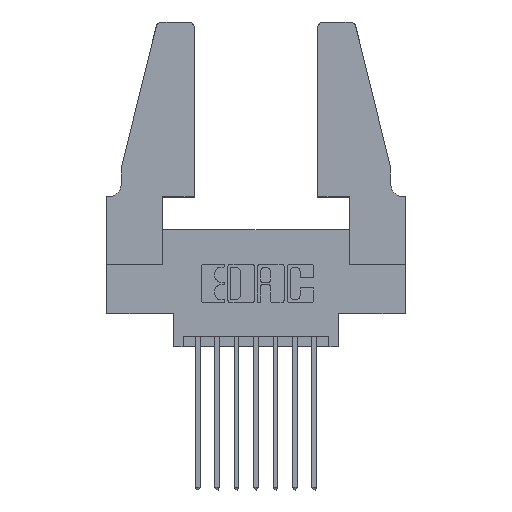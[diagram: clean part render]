
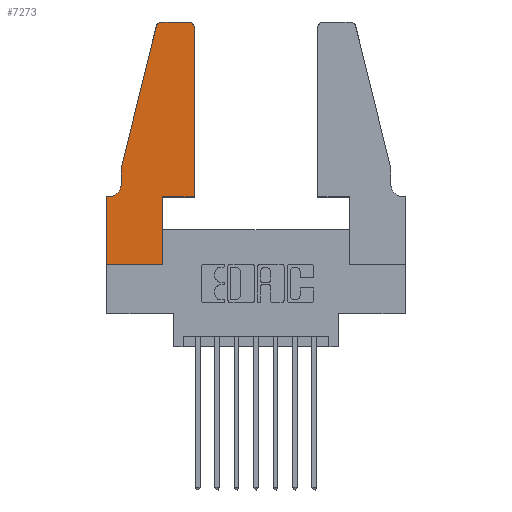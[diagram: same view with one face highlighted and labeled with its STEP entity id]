
A CAD part, top view. The second image highlights one B-rep face of the part: STEP entity #7273.
In plain terms, the highlighted planar face has unit normal (0, 0, 1).
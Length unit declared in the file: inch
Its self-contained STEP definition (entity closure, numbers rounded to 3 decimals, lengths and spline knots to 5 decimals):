
#127 = EDGE_CURVE ( 'NONE', #12425, #11473, #196, .T. ) ;
#196 = LINE ( 'NONE', #6369, #12167 ) ;
#222 = AXIS2_PLACEMENT_3D ( 'NONE', #2754, #9478, #3742 ) ;
#242 = ORIENTED_EDGE ( 'NONE', *, *, #4428, .T. ) ;
#243 = CARTESIAN_POINT ( 'NONE',  ( 0., 0., 0.37 ) ) ;
#320 = CARTESIAN_POINT ( 'NONE',  ( 0.4505, 1.22, 0.37 ) ) ;
#389 = VERTEX_POINT ( 'NONE', #8444 ) ;
#683 = AXIS2_PLACEMENT_3D ( 'NONE', #7033, #11003, #5285 ) ;
#703 = DIRECTION ( 'NONE',  ( 0., 0., 1. ) ) ;
#726 = DIRECTION ( 'NONE',  ( -1., 0., 0. ) ) ;
#763 = LINE ( 'NONE', #7989, #8555 ) ;
#957 = EDGE_CURVE ( 'NONE', #11473, #7178, #2600, .T. ) ;
#1103 = ORIENTED_EDGE ( 'NONE', *, *, #127, .T. ) ;
#1180 = DIRECTION ( 'NONE',  ( -1., 0., 0. ) ) ;
#1205 = DIRECTION ( 'NONE',  ( 0., -1., 0. ) ) ;
#1503 = LINE ( 'NONE', #6315, #8959 ) ;
#1654 = VECTOR ( 'NONE', #5537, 39.37008 ) ;
#1711 = CARTESIAN_POINT ( 'NONE',  ( 0.0055, 0.35, 0.37 ) ) ;
#1788 = CARTESIAN_POINT ( 'NONE',  ( 0.2865, 0.35, 0.37 ) ) ;
#1883 = CARTESIAN_POINT ( 'NONE',  ( 0.4505, 0.35, 0.37 ) ) ;
#2232 = VECTOR ( 'NONE', #12325, 39.37008 ) ;
#2252 = CARTESIAN_POINT ( 'NONE',  ( 0., 0., 0.37 ) ) ;
#2409 = CARTESIAN_POINT ( 'NONE',  ( 0., 0.35, 0.37 ) ) ;
#2600 = LINE ( 'NONE', #5338, #1654 ) ;
#2636 = ORIENTED_EDGE ( 'NONE', *, *, #8829, .T. ) ;
#2751 = CARTESIAN_POINT ( 'NONE',  ( 0.0755, 0.5, 0.37 ) ) ;
#2754 = CARTESIAN_POINT ( 'NONE',  ( 0.4205, 1.22, 0.37 ) ) ;
#2934 = VECTOR ( 'NONE', #3273, 39.37008 ) ;
#3187 = EDGE_CURVE ( 'NONE', #7178, #6817, #763, .T. ) ;
#3273 = DIRECTION ( 'NONE',  ( -0.239, -0.971, 0. ) ) ;
#3488 = VERTEX_POINT ( 'NONE', #11313 ) ;
#3649 = VERTEX_POINT ( 'NONE', #243 ) ;
#3742 = DIRECTION ( 'NONE',  ( 1., 0., 0. ) ) ;
#3985 = CIRCLE ( 'NONE', #6483, 0.03 ) ;
#4185 = CARTESIAN_POINT ( 'NONE',  ( 0.0755, 0.5, 0.37 ) ) ;
#4303 = PLANE ( 'NONE',  #683 ) ;
#4428 = EDGE_CURVE ( 'NONE', #389, #3488, #3985, .T. ) ;
#4557 = CARTESIAN_POINT ( 'NONE',  ( 0.0755, 0.42, 0.37 ) ) ;
#4582 = LINE ( 'NONE', #2252, #9116 ) ;
#4612 = EDGE_CURVE ( 'NONE', #12390, #3649, #1503, .T. ) ;
#4676 = ORIENTED_EDGE ( 'NONE', *, *, #10158, .T. ) ;
#4779 = ORIENTED_EDGE ( 'NONE', *, *, #3187, .T. ) ;
#5044 = ORIENTED_EDGE ( 'NONE', *, *, #5746, .T. ) ;
#5285 = DIRECTION ( 'NONE',  ( 1., 0., 0. ) ) ;
#5332 = CARTESIAN_POINT ( 'NONE',  ( 0.284, 1.22, 0.37 ) ) ;
#5338 = CARTESIAN_POINT ( 'NONE',  ( 0.4505, 0.35, 0.37 ) ) ;
#5505 = LINE ( 'NONE', #4185, #2934 ) ;
#5537 = DIRECTION ( 'NONE',  ( 1., 0., 0. ) ) ;
#5682 = ORIENTED_EDGE ( 'NONE', *, *, #4612, .T. ) ;
#5746 = EDGE_CURVE ( 'NONE', #9139, #10770, #11568, .T. ) ;
#5865 = FACE_OUTER_BOUND ( 'NONE', #8997, .T. ) ;
#6110 = ORIENTED_EDGE ( 'NONE', *, *, #10468, .T. ) ;
#6315 = CARTESIAN_POINT ( 'NONE',  ( 0., 0., 0.37 ) ) ;
#6369 = CARTESIAN_POINT ( 'NONE',  ( 0.2865, 0.35, 0.37 ) ) ;
#6483 = AXIS2_PLACEMENT_3D ( 'NONE', #5332, #703, #10386 ) ;
#6590 = DIRECTION ( 'NONE',  ( 0., 0., -1. ) ) ;
#6817 = VERTEX_POINT ( 'NONE', #320 ) ;
#7033 = CARTESIAN_POINT ( 'NONE',  ( 0., 0.35, 0.37 ) ) ;
#7052 = EDGE_CURVE ( 'NONE', #6817, #12156, #12406, .T. ) ;
#7080 = EDGE_CURVE ( 'NONE', #10770, #12390, #12118, .T. ) ;
#7178 = VERTEX_POINT ( 'NONE', #1883 ) ;
#7273 = ADVANCED_FACE ( 'NONE', ( #5865 ), #4303, .T. ) ;
#7989 = CARTESIAN_POINT ( 'NONE',  ( 0.4505, 0.35, 0.37 ) ) ;
#8444 = CARTESIAN_POINT ( 'NONE',  ( 0.284, 1.25, 0.37 ) ) ;
#8552 = CARTESIAN_POINT ( 'NONE',  ( 0.0755, 0.35, 0.37 ) ) ;
#8555 = VECTOR ( 'NONE', #10360, 39.37008 ) ;
#8829 = EDGE_CURVE ( 'NONE', #12156, #389, #11228, .T. ) ;
#8959 = VECTOR ( 'NONE', #1205, 39.37008 ) ;
#8997 = EDGE_LOOP ( 'NONE', ( #2636, #242, #6110, #11197, #5044, #10147, #5682, #4676, #1103, #11805, #4779, #10378 ) ) ;
#9116 = VECTOR ( 'NONE', #9980, 39.37008 ) ;
#9139 = VERTEX_POINT ( 'NONE', #4557 ) ;
#9463 = CARTESIAN_POINT ( 'NONE',  ( 0.0755, 0.5, 0.37 ) ) ;
#9477 = DIRECTION ( 'NONE',  ( 0., -1., 0. ) ) ;
#9478 = DIRECTION ( 'NONE',  ( 0., 0., 1. ) ) ;
#9823 = VERTEX_POINT ( 'NONE', #9463 ) ;
#9980 = DIRECTION ( 'NONE',  ( 1., 0., 0. ) ) ;
#10136 = CARTESIAN_POINT ( 'NONE',  ( 0.2865, 0., 0.37 ) ) ;
#10147 = ORIENTED_EDGE ( 'NONE', *, *, #7080, .T. ) ;
#10158 = EDGE_CURVE ( 'NONE', #3649, #12425, #4582, .T. ) ;
#10360 = DIRECTION ( 'NONE',  ( 0., 1., 0. ) ) ;
#10378 = ORIENTED_EDGE ( 'NONE', *, *, #7052, .T. ) ;
#10386 = DIRECTION ( 'NONE',  ( 1., 0., 0. ) ) ;
#10468 = EDGE_CURVE ( 'NONE', #3488, #9823, #5505, .T. ) ;
#10569 = AXIS2_PLACEMENT_3D ( 'NONE', #12272, #6590, #726 ) ;
#10650 = CARTESIAN_POINT ( 'NONE',  ( 0.4205, 1.25, 0.37 ) ) ;
#10770 = VERTEX_POINT ( 'NONE', #1711 ) ;
#10801 = EDGE_CURVE ( 'NONE', #9823, #9139, #11458, .T. ) ;
#10812 = CARTESIAN_POINT ( 'NONE',  ( 0.2605, 1.25, 0.37 ) ) ;
#10911 = VECTOR ( 'NONE', #1180, 39.37008 ) ;
#11003 = DIRECTION ( 'NONE',  ( 0., 0., 1. ) ) ;
#11197 = ORIENTED_EDGE ( 'NONE', *, *, #10801, .T. ) ;
#11228 = LINE ( 'NONE', #10812, #10911 ) ;
#11313 = CARTESIAN_POINT ( 'NONE',  ( 0.25487, 1.22718, 0.37 ) ) ;
#11458 = LINE ( 'NONE', #2751, #11754 ) ;
#11473 = VERTEX_POINT ( 'NONE', #1788 ) ;
#11568 = CIRCLE ( 'NONE', #10569, 0.07 ) ;
#11754 = VECTOR ( 'NONE', #9477, 39.37008 ) ;
#11805 = ORIENTED_EDGE ( 'NONE', *, *, #957, .T. ) ;
#12058 = DIRECTION ( 'NONE',  ( 0., 1., 0. ) ) ;
#12118 = LINE ( 'NONE', #8552, #2232 ) ;
#12156 = VERTEX_POINT ( 'NONE', #10650 ) ;
#12167 = VECTOR ( 'NONE', #12058, 39.37008 ) ;
#12272 = CARTESIAN_POINT ( 'NONE',  ( 0.0055, 0.42, 0.37 ) ) ;
#12325 = DIRECTION ( 'NONE',  ( -1., 0., 0. ) ) ;
#12390 = VERTEX_POINT ( 'NONE', #2409 ) ;
#12406 = CIRCLE ( 'NONE', #222, 0.03 ) ;
#12425 = VERTEX_POINT ( 'NONE', #10136 ) ;
